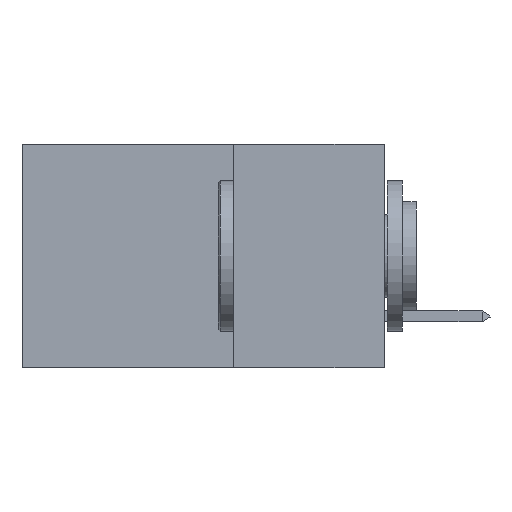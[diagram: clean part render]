
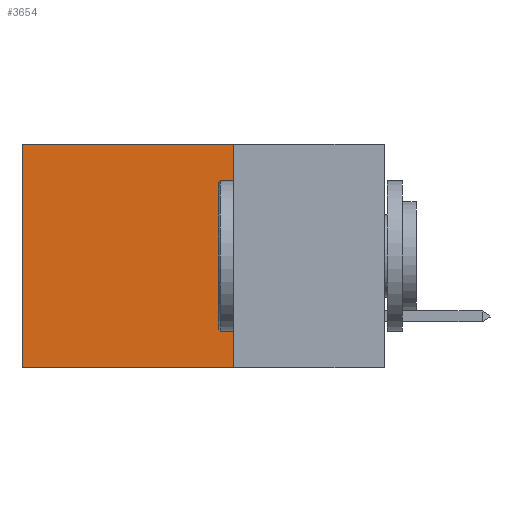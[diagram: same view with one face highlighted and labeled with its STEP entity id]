
A CAD part, left-side view. The second image highlights one B-rep face of the part: STEP entity #3654.
In plain terms, the highlighted planar face has unit normal (-1, 0, 0).
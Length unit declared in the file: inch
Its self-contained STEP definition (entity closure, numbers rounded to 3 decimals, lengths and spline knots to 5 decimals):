
#518 = DIRECTION ( 'NONE',  ( 0., 0., -1. ) ) ;
#607 = CARTESIAN_POINT ( 'NONE',  ( 0.2875, 0.25, -0.37 ) ) ;
#1076 = LINE ( 'NONE', #607, #11688 ) ;
#1378 = VERTEX_POINT ( 'NONE', #26366 ) ;
#3654 = ADVANCED_FACE ( 'NONE', ( #5937 ), #9564, .F. ) ;
#4413 = LINE ( 'NONE', #7131, #14627 ) ;
#4612 = ORIENTED_EDGE ( 'NONE', *, *, #22310, .T. ) ;
#5397 = ORIENTED_EDGE ( 'NONE', *, *, #22974, .F. ) ;
#5937 = FACE_OUTER_BOUND ( 'NONE', #11282, .T. ) ;
#6708 = ORIENTED_EDGE ( 'NONE', *, *, #13437, .T. ) ;
#7131 = CARTESIAN_POINT ( 'NONE',  ( 0.2875, 0.25, 0. ) ) ;
#7225 = LINE ( 'NONE', #8695, #14634 ) ;
#8695 = CARTESIAN_POINT ( 'NONE',  ( 0.2875, 0.25, 0. ) ) ;
#9564 = PLANE ( 'NONE',  #28423 ) ;
#9565 = VERTEX_POINT ( 'NONE', #13207 ) ;
#10851 = VECTOR ( 'NONE', #518, 39.37008 ) ;
#11282 = EDGE_LOOP ( 'NONE', ( #6708, #13145, #5397, #4612 ) ) ;
#11609 = VERTEX_POINT ( 'NONE', #28496 ) ;
#11688 = VECTOR ( 'NONE', #23449, 39.37008 ) ;
#13145 = ORIENTED_EDGE ( 'NONE', *, *, #25101, .F. ) ;
#13207 = CARTESIAN_POINT ( 'NONE',  ( 0.2875, 0.25, -0.37 ) ) ;
#13437 = EDGE_CURVE ( 'NONE', #1378, #11609, #22827, .T. ) ;
#14627 = VECTOR ( 'NONE', #18883, 39.37008 ) ;
#14634 = VECTOR ( 'NONE', #20020, 39.37008 ) ;
#18500 = DIRECTION ( 'NONE',  ( 1., 0., 0. ) ) ;
#18883 = DIRECTION ( 'NONE',  ( 0., 1., 0. ) ) ;
#19382 = VERTEX_POINT ( 'NONE', #23024 ) ;
#20020 = DIRECTION ( 'NONE',  ( 0., 0., -1. ) ) ;
#22310 = EDGE_CURVE ( 'NONE', #19382, #1378, #4413, .T. ) ;
#22664 = CARTESIAN_POINT ( 'NONE',  ( 0.2875, 0.25, 0. ) ) ;
#22827 = LINE ( 'NONE', #24326, #10851 ) ;
#22974 = EDGE_CURVE ( 'NONE', #19382, #9565, #7225, .T. ) ;
#23024 = CARTESIAN_POINT ( 'NONE',  ( 0.2875, 0.25, 0. ) ) ;
#23449 = DIRECTION ( 'NONE',  ( 0., 1., 0. ) ) ;
#24326 = CARTESIAN_POINT ( 'NONE',  ( 0.2875, 0.6, 0. ) ) ;
#25038 = DIRECTION ( 'NONE',  ( 0., 0., -1. ) ) ;
#25101 = EDGE_CURVE ( 'NONE', #9565, #11609, #1076, .T. ) ;
#26366 = CARTESIAN_POINT ( 'NONE',  ( 0.2875, 0.6, 0. ) ) ;
#28423 = AXIS2_PLACEMENT_3D ( 'NONE', #22664, #18500, #25038 ) ;
#28496 = CARTESIAN_POINT ( 'NONE',  ( 0.2875, 0.6, -0.37 ) ) ;
